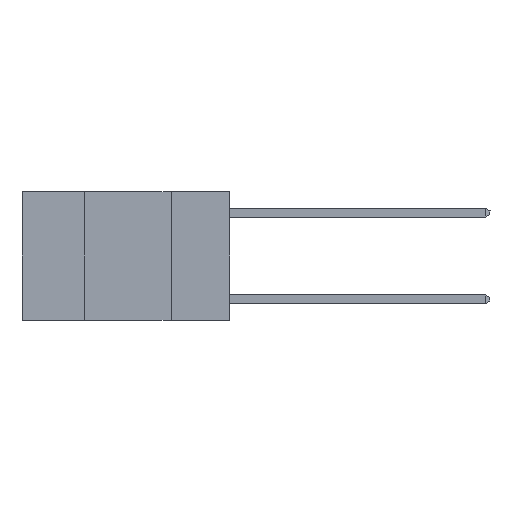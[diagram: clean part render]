
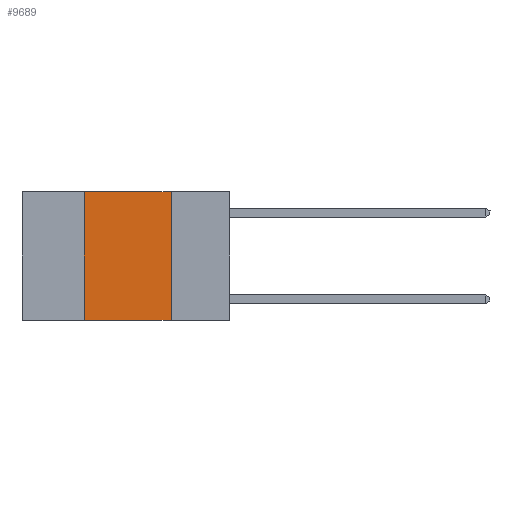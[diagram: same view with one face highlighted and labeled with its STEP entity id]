
A CAD part, left-side view. The second image highlights one B-rep face of the part: STEP entity #9689.
In plain terms, the highlighted planar face has unit normal (-1, 0, 0).
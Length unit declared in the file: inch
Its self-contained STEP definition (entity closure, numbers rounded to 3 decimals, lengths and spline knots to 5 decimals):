
#102 = DIRECTION ( 'NONE',  ( 0., -1., 0. ) ) ;
#469 = CARTESIAN_POINT ( 'NONE',  ( 0., 0.17, 0. ) ) ;
#590 = DIRECTION ( 'NONE',  ( 0., 0., -1. ) ) ;
#1008 = CARTESIAN_POINT ( 'NONE',  ( 0., 0.6, -0.37 ) ) ;
#2174 = LINE ( 'NONE', #469, #11483 ) ;
#2502 = LINE ( 'NONE', #1008, #9426 ) ;
#2774 = CARTESIAN_POINT ( 'NONE',  ( 0., 0.17, -0.37 ) ) ;
#2846 = CARTESIAN_POINT ( 'NONE',  ( 0., 0.17, 0. ) ) ;
#3345 = VERTEX_POINT ( 'NONE', #4204 ) ;
#4204 = CARTESIAN_POINT ( 'NONE',  ( 0., 0.42, -0.37 ) ) ;
#4770 = ORIENTED_EDGE ( 'NONE', *, *, #4937, .T. ) ;
#4937 = EDGE_CURVE ( 'NONE', #3345, #5558, #2502, .T. ) ;
#5029 = ORIENTED_EDGE ( 'NONE', *, *, #7540, .F. ) ;
#5041 = EDGE_LOOP ( 'NONE', ( #5029, #11032, #11212, #4770 ) ) ;
#5116 = CARTESIAN_POINT ( 'NONE',  ( 0., 0.6, 0. ) ) ;
#5558 = VERTEX_POINT ( 'NONE', #2774 ) ;
#5646 = EDGE_CURVE ( 'NONE', #3345, #10983, #7448, .T. ) ;
#5892 = DIRECTION ( 'NONE',  ( 0., -1., 0. ) ) ;
#5961 = FACE_OUTER_BOUND ( 'NONE', #5041, .T. ) ;
#6019 = DIRECTION ( 'NONE',  ( 1., 0., 0. ) ) ;
#6935 = LINE ( 'NONE', #10363, #9030 ) ;
#7157 = VECTOR ( 'NONE', #11004, 39.37008 ) ;
#7448 = LINE ( 'NONE', #7453, #7157 ) ;
#7453 = CARTESIAN_POINT ( 'NONE',  ( 0., 0.42, 0. ) ) ;
#7540 = EDGE_CURVE ( 'NONE', #9410, #5558, #2174, .T. ) ;
#8648 = DIRECTION ( 'NONE',  ( 0., 0., -1. ) ) ;
#9030 = VECTOR ( 'NONE', #5892, 39.37008 ) ;
#9410 = VERTEX_POINT ( 'NONE', #2846 ) ;
#9426 = VECTOR ( 'NONE', #102, 39.37008 ) ;
#9580 = CARTESIAN_POINT ( 'NONE',  ( 0., 0.42, 0. ) ) ;
#9689 = ADVANCED_FACE ( 'NONE', ( #5961 ), #10499, .F. ) ;
#10256 = EDGE_CURVE ( 'NONE', #10983, #9410, #6935, .T. ) ;
#10363 = CARTESIAN_POINT ( 'NONE',  ( 0., 0.6, 0. ) ) ;
#10499 = PLANE ( 'NONE',  #10982 ) ;
#10982 = AXIS2_PLACEMENT_3D ( 'NONE', #5116, #6019, #590 ) ;
#10983 = VERTEX_POINT ( 'NONE', #9580 ) ;
#11004 = DIRECTION ( 'NONE',  ( 0., 0., 1. ) ) ;
#11032 = ORIENTED_EDGE ( 'NONE', *, *, #10256, .F. ) ;
#11212 = ORIENTED_EDGE ( 'NONE', *, *, #5646, .F. ) ;
#11483 = VECTOR ( 'NONE', #8648, 39.37008 ) ;
